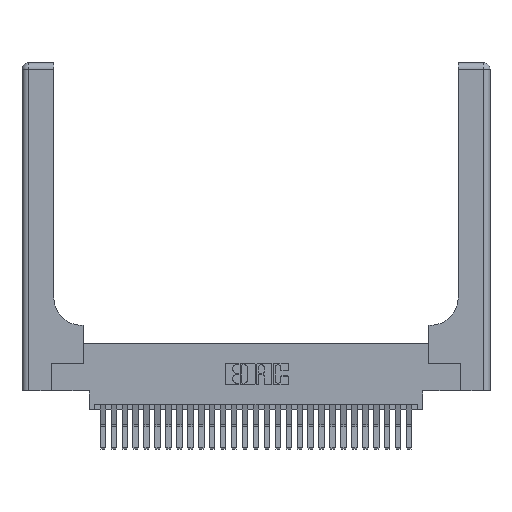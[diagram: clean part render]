
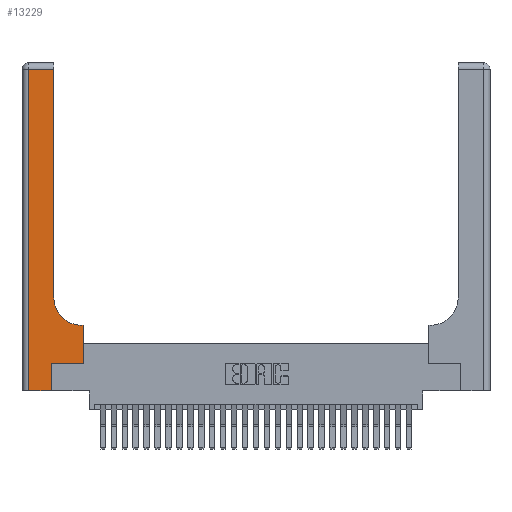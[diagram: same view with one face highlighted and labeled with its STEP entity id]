
A CAD part, top view. The second image highlights one B-rep face of the part: STEP entity #13229.
In plain terms, the highlighted planar face has unit normal (0, 0, 1).
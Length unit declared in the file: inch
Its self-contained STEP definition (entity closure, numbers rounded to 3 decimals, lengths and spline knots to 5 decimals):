
#232 = CARTESIAN_POINT ( 'NONE',  ( 0., 0., 0.37 ) ) ;
#1705 = VECTOR ( 'NONE', #26951, 39.37008 ) ;
#2901 = LINE ( 'NONE', #29135, #7613 ) ;
#3167 = LINE ( 'NONE', #232, #20865 ) ;
#3261 = VECTOR ( 'NONE', #17687, 39.37008 ) ;
#3944 = VERTEX_POINT ( 'NONE', #28173 ) ;
#4679 = ORIENTED_EDGE ( 'NONE', *, *, #9722, .T. ) ;
#5078 = EDGE_CURVE ( 'NONE', #3944, #9699, #23511, .T. ) ;
#5869 = CARTESIAN_POINT ( 'NONE',  ( 0., 3., 0.37 ) ) ;
#5930 = VERTEX_POINT ( 'NONE', #29711 ) ;
#7363 = CIRCLE ( 'NONE', #15508, 0.25 ) ;
#7613 = VECTOR ( 'NONE', #10902, 39.37008 ) ;
#7876 = PLANE ( 'NONE',  #8302 ) ;
#8068 = VECTOR ( 'NONE', #21995, 39.37008 ) ;
#8105 = EDGE_CURVE ( 'NONE', #27371, #3944, #28077, .T. ) ;
#8302 = AXIS2_PLACEMENT_3D ( 'NONE', #5869, #19353, #24128 ) ;
#8516 = ORIENTED_EDGE ( 'NONE', *, *, #8105, .T. ) ;
#8559 = ORIENTED_EDGE ( 'NONE', *, *, #5078, .T. ) ;
#8780 = CARTESIAN_POINT ( 'NONE',  ( 0., 2.94, 0.37 ) ) ;
#9089 = EDGE_CURVE ( 'NONE', #19146, #10372, #23331, .T. ) ;
#9441 = LINE ( 'NONE', #20760, #17725 ) ;
#9699 = VERTEX_POINT ( 'NONE', #20163 ) ;
#9722 = EDGE_CURVE ( 'NONE', #10372, #24686, #20002, .T. ) ;
#9732 = DIRECTION ( 'NONE',  ( 0., 0., -1. ) ) ;
#9903 = EDGE_CURVE ( 'NONE', #24686, #5930, #7363, .T. ) ;
#10025 = FACE_OUTER_BOUND ( 'NONE', #21482, .T. ) ;
#10372 = VERTEX_POINT ( 'NONE', #20243 ) ;
#10902 = DIRECTION ( 'NONE',  ( 0., 1., 0. ) ) ;
#12443 = ORIENTED_EDGE ( 'NONE', *, *, #23988, .T. ) ;
#13229 = ADVANCED_FACE ( 'NONE', ( #10025 ), #7876, .F. ) ;
#13457 = DIRECTION ( 'NONE',  ( 1., 0., 0. ) ) ;
#13850 = DIRECTION ( 'NONE',  ( -1., 0., 0. ) ) ;
#14271 = CARTESIAN_POINT ( 'NONE',  ( 0.5415, 0.85, 0.37 ) ) ;
#15125 = CARTESIAN_POINT ( 'NONE',  ( 0.2915, 2.94, 0.37 ) ) ;
#15508 = AXIS2_PLACEMENT_3D ( 'NONE', #14271, #9732, #13457 ) ;
#15788 = ORIENTED_EDGE ( 'NONE', *, *, #9089, .T. ) ;
#16232 = DIRECTION ( 'NONE',  ( 1., 0., 0. ) ) ;
#16577 = CARTESIAN_POINT ( 'NONE',  ( 0.269, 0.25, 0.37 ) ) ;
#17497 = VECTOR ( 'NONE', #13850, 39.37008 ) ;
#17687 = DIRECTION ( 'NONE',  ( 0., -1., 0. ) ) ;
#17725 = VECTOR ( 'NONE', #23088, 39.37008 ) ;
#18822 = CARTESIAN_POINT ( 'NONE',  ( 0.5585, 0.25, 0.37 ) ) ;
#19146 = VERTEX_POINT ( 'NONE', #18822 ) ;
#19353 = DIRECTION ( 'NONE',  ( 0., 0., -1. ) ) ;
#19670 = CARTESIAN_POINT ( 'NONE',  ( 0.5585, 0.25, 0.37 ) ) ;
#20002 = LINE ( 'NONE', #20969, #17497 ) ;
#20096 = CARTESIAN_POINT ( 'NONE',  ( 0.06, 3., 0.37 ) ) ;
#20163 = CARTESIAN_POINT ( 'NONE',  ( 0.06, 0., 0.37 ) ) ;
#20243 = CARTESIAN_POINT ( 'NONE',  ( 0.5585, 0.6, 0.37 ) ) ;
#20611 = CARTESIAN_POINT ( 'NONE',  ( 0.269, 0., 0.37 ) ) ;
#20760 = CARTESIAN_POINT ( 'NONE',  ( 0.2915, 3., 0.37 ) ) ;
#20865 = VECTOR ( 'NONE', #16232, 39.37008 ) ;
#20969 = CARTESIAN_POINT ( 'NONE',  ( 0.2915, 0.6, 0.37 ) ) ;
#21069 = ORIENTED_EDGE ( 'NONE', *, *, #23447, .T. ) ;
#21073 = LINE ( 'NONE', #16577, #8068 ) ;
#21393 = EDGE_CURVE ( 'NONE', #9699, #27591, #3167, .T. ) ;
#21482 = EDGE_LOOP ( 'NONE', ( #12443, #8516, #8559, #26335, #23663, #21069, #15788, #4679, #23569 ) ) ;
#21636 = CARTESIAN_POINT ( 'NONE',  ( 0.5415, 0.6, 0.37 ) ) ;
#21995 = DIRECTION ( 'NONE',  ( 1., 0., 0. ) ) ;
#23088 = DIRECTION ( 'NONE',  ( 0., 1., 0. ) ) ;
#23331 = LINE ( 'NONE', #19670, #28371 ) ;
#23447 = EDGE_CURVE ( 'NONE', #28291, #19146, #21073, .T. ) ;
#23511 = LINE ( 'NONE', #20096, #3261 ) ;
#23569 = ORIENTED_EDGE ( 'NONE', *, *, #9903, .T. ) ;
#23663 = ORIENTED_EDGE ( 'NONE', *, *, #24214, .T. ) ;
#23988 = EDGE_CURVE ( 'NONE', #5930, #27371, #9441, .T. ) ;
#24128 = DIRECTION ( 'NONE',  ( -1., 0., 0. ) ) ;
#24214 = EDGE_CURVE ( 'NONE', #27591, #28291, #2901, .T. ) ;
#24252 = DIRECTION ( 'NONE',  ( 0., 1., 0. ) ) ;
#24686 = VERTEX_POINT ( 'NONE', #21636 ) ;
#25426 = CARTESIAN_POINT ( 'NONE',  ( 0.269, 0.25, 0.37 ) ) ;
#26335 = ORIENTED_EDGE ( 'NONE', *, *, #21393, .T. ) ;
#26951 = DIRECTION ( 'NONE',  ( -1., 0., 0. ) ) ;
#27371 = VERTEX_POINT ( 'NONE', #15125 ) ;
#27591 = VERTEX_POINT ( 'NONE', #20611 ) ;
#28077 = LINE ( 'NONE', #8780, #1705 ) ;
#28173 = CARTESIAN_POINT ( 'NONE',  ( 0.06, 2.94, 0.37 ) ) ;
#28291 = VERTEX_POINT ( 'NONE', #25426 ) ;
#28371 = VECTOR ( 'NONE', #24252, 39.37008 ) ;
#29135 = CARTESIAN_POINT ( 'NONE',  ( 0.269, 0., 0.37 ) ) ;
#29711 = CARTESIAN_POINT ( 'NONE',  ( 0.2915, 0.85, 0.37 ) ) ;
